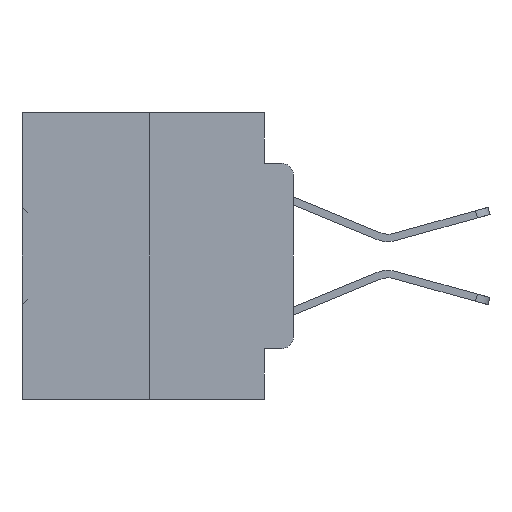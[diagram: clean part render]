
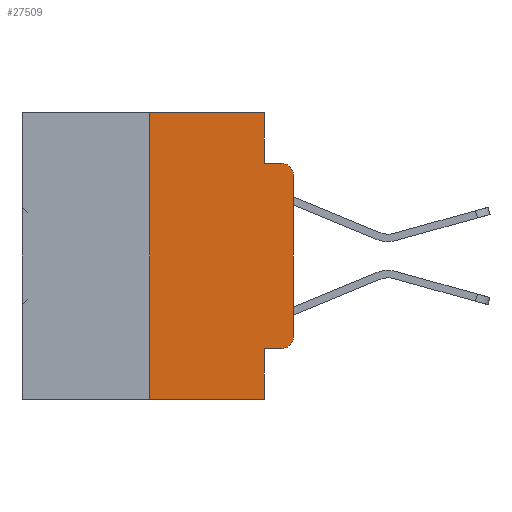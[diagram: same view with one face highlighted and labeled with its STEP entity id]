
A CAD part, left-side view. The second image highlights one B-rep face of the part: STEP entity #27509.
In plain terms, the highlighted planar face has unit normal (-1, 0, 0).
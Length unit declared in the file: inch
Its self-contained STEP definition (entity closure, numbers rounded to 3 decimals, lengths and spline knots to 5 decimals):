
#303 = CARTESIAN_POINT ( 'NONE',  ( 0., 0.473, -0.5 ) ) ;
#513 = VERTEX_POINT ( 'NONE', #27313 ) ;
#673 = CARTESIAN_POINT ( 'NONE',  ( 0., 0.25, 0. ) ) ;
#717 = ORIENTED_EDGE ( 'NONE', *, *, #29389, .F. ) ;
#874 = CARTESIAN_POINT ( 'NONE',  ( 0., 0.051, 0. ) ) ;
#1367 = DIRECTION ( 'NONE',  ( 0., 0., 1. ) ) ;
#2021 = EDGE_CURVE ( 'NONE', #513, #26204, #29600, .T. ) ;
#4090 = EDGE_CURVE ( 'NONE', #15881, #15574, #36433, .T. ) ;
#4099 = CARTESIAN_POINT ( 'NONE',  ( 0., 0., -0.1085 ) ) ;
#4382 = CARTESIAN_POINT ( 'NONE',  ( 0., 0.473, 0. ) ) ;
#5366 = DIRECTION ( 'NONE',  ( 0., 0., -1. ) ) ;
#5858 = CARTESIAN_POINT ( 'NONE',  ( 0., 0., -0.3915 ) ) ;
#5866 = LINE ( 'NONE', #303, #27303 ) ;
#6358 = EDGE_CURVE ( 'NONE', #32419, #15574, #7199, .T. ) ;
#7179 = LINE ( 'NONE', #874, #32295 ) ;
#7199 = CIRCLE ( 'NONE', #18476, 0.02 ) ;
#7299 = LINE ( 'NONE', #673, #12323 ) ;
#7555 = CARTESIAN_POINT ( 'NONE',  ( 0., 0.051, 0. ) ) ;
#7842 = CARTESIAN_POINT ( 'NONE',  ( 0., 0.051, -0.4115 ) ) ;
#7857 = CARTESIAN_POINT ( 'NONE',  ( 0., 0.051, -0.5 ) ) ;
#7962 = PLANE ( 'NONE',  #8562 ) ;
#8184 = VECTOR ( 'NONE', #19711, 39.37008 ) ;
#8562 = AXIS2_PLACEMENT_3D ( 'NONE', #36402, #28200, #5366 ) ;
#9136 = EDGE_CURVE ( 'NONE', #26204, #32419, #30774, .T. ) ;
#9679 = VERTEX_POINT ( 'NONE', #19560 ) ;
#11607 = DIRECTION ( 'NONE',  ( 0., -1., 0. ) ) ;
#12095 = CARTESIAN_POINT ( 'NONE',  ( 0., 0.02, -0.3915 ) ) ;
#12323 = VECTOR ( 'NONE', #1367, 39.37008 ) ;
#12939 = DIRECTION ( 'NONE',  ( 0., 0., -1. ) ) ;
#13619 = VERTEX_POINT ( 'NONE', #27707 ) ;
#13662 = CARTESIAN_POINT ( 'NONE',  ( 0., 0., 0. ) ) ;
#14634 = VERTEX_POINT ( 'NONE', #17375 ) ;
#15139 = DIRECTION ( 'NONE',  ( 0., -1., 0. ) ) ;
#15439 = ORIENTED_EDGE ( 'NONE', *, *, #9136, .T. ) ;
#15574 = VERTEX_POINT ( 'NONE', #34341 ) ;
#15881 = VERTEX_POINT ( 'NONE', #22228 ) ;
#17103 = ORIENTED_EDGE ( 'NONE', *, *, #32148, .T. ) ;
#17375 = CARTESIAN_POINT ( 'NONE',  ( 0., 0.25, 0. ) ) ;
#17566 = VECTOR ( 'NONE', #15139, 39.37008 ) ;
#18476 = AXIS2_PLACEMENT_3D ( 'NONE', #32751, #24386, #30140 ) ;
#19440 = EDGE_CURVE ( 'NONE', #13619, #15881, #33014, .T. ) ;
#19493 = DIRECTION ( 'NONE',  ( 0., -1., 0. ) ) ;
#19560 = CARTESIAN_POINT ( 'NONE',  ( 0., 0.25, -0.5 ) ) ;
#19711 = DIRECTION ( 'NONE',  ( 0., -1., 0. ) ) ;
#20488 = CARTESIAN_POINT ( 'NONE',  ( 0., 0.051, -0.4115 ) ) ;
#20570 = ORIENTED_EDGE ( 'NONE', *, *, #31932, .F. ) ;
#22228 = CARTESIAN_POINT ( 'NONE',  ( 0., 0.051, -0.0885 ) ) ;
#23074 = ORIENTED_EDGE ( 'NONE', *, *, #2021, .T. ) ;
#23953 = EDGE_LOOP ( 'NONE', ( #15439, #31545, #34537, #30050, #717, #20570, #25438, #36505, #17103, #23074 ) ) ;
#24386 = DIRECTION ( 'NONE',  ( -1., 0., 0. ) ) ;
#24531 = VECTOR ( 'NONE', #27969, 39.37008 ) ;
#25230 = VERTEX_POINT ( 'NONE', #7857 ) ;
#25438 = ORIENTED_EDGE ( 'NONE', *, *, #36225, .T. ) ;
#25775 = VECTOR ( 'NONE', #19493, 39.37008 ) ;
#25806 = CARTESIAN_POINT ( 'NONE',  ( 0., 0.051, -0.0885 ) ) ;
#25920 = EDGE_CURVE ( 'NONE', #33867, #25230, #7179, .T. ) ;
#26204 = VERTEX_POINT ( 'NONE', #5858 ) ;
#27211 = LINE ( 'NONE', #4382, #17566 ) ;
#27216 = AXIS2_PLACEMENT_3D ( 'NONE', #12095, #29884, #35475 ) ;
#27303 = VECTOR ( 'NONE', #11607, 39.37008 ) ;
#27313 = CARTESIAN_POINT ( 'NONE',  ( 0., 0.02, -0.4115 ) ) ;
#27419 = DIRECTION ( 'NONE',  ( 0., 0., -1. ) ) ;
#27509 = ADVANCED_FACE ( 'NONE', ( #30811 ), #7962, .F. ) ;
#27707 = CARTESIAN_POINT ( 'NONE',  ( 0., 0.051, 0. ) ) ;
#27969 = DIRECTION ( 'NONE',  ( 0., 0., 1. ) ) ;
#28200 = DIRECTION ( 'NONE',  ( 1., 0., 0. ) ) ;
#29389 = EDGE_CURVE ( 'NONE', #14634, #13619, #27211, .T. ) ;
#29600 = CIRCLE ( 'NONE', #27216, 0.02 ) ;
#29652 = VECTOR ( 'NONE', #27419, 39.37008 ) ;
#29884 = DIRECTION ( 'NONE',  ( -1., 0., 0. ) ) ;
#30050 = ORIENTED_EDGE ( 'NONE', *, *, #19440, .F. ) ;
#30140 = DIRECTION ( 'NONE',  ( 0., 0., -1. ) ) ;
#30774 = LINE ( 'NONE', #13662, #24531 ) ;
#30811 = FACE_OUTER_BOUND ( 'NONE', #23953, .T. ) ;
#31545 = ORIENTED_EDGE ( 'NONE', *, *, #6358, .T. ) ;
#31932 = EDGE_CURVE ( 'NONE', #9679, #14634, #7299, .T. ) ;
#32148 = EDGE_CURVE ( 'NONE', #33867, #513, #34027, .T. ) ;
#32295 = VECTOR ( 'NONE', #12939, 39.37008 ) ;
#32419 = VERTEX_POINT ( 'NONE', #4099 ) ;
#32751 = CARTESIAN_POINT ( 'NONE',  ( 0., 0.02, -0.1085 ) ) ;
#33014 = LINE ( 'NONE', #7555, #29652 ) ;
#33867 = VERTEX_POINT ( 'NONE', #20488 ) ;
#34027 = LINE ( 'NONE', #7842, #8184 ) ;
#34341 = CARTESIAN_POINT ( 'NONE',  ( 0., 0.02, -0.0885 ) ) ;
#34537 = ORIENTED_EDGE ( 'NONE', *, *, #4090, .F. ) ;
#35475 = DIRECTION ( 'NONE',  ( 0., 0., -1. ) ) ;
#36225 = EDGE_CURVE ( 'NONE', #9679, #25230, #5866, .T. ) ;
#36402 = CARTESIAN_POINT ( 'NONE',  ( 0., 0.473, 0. ) ) ;
#36433 = LINE ( 'NONE', #25806, #25775 ) ;
#36505 = ORIENTED_EDGE ( 'NONE', *, *, #25920, .F. ) ;
